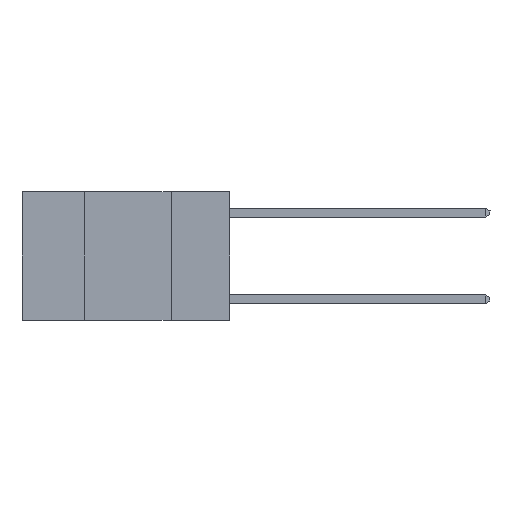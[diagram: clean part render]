
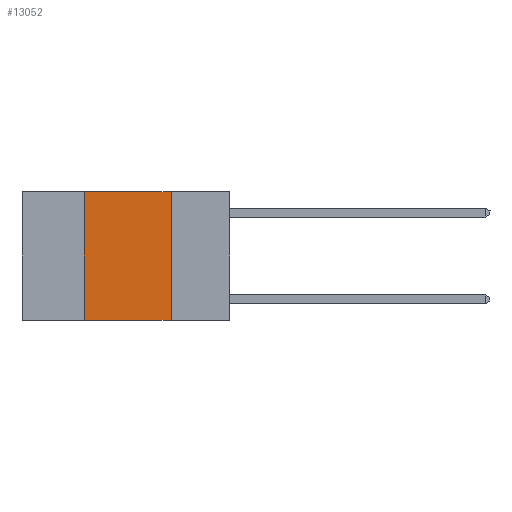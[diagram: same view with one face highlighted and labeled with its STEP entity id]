
A CAD part, left-side view. The second image highlights one B-rep face of the part: STEP entity #13052.
In plain terms, the highlighted planar face has unit normal (-1, 0, 0).
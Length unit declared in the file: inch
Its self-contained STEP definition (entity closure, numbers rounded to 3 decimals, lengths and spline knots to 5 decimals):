
#58 = VERTEX_POINT ( 'NONE', #12671 ) ;
#688 = VECTOR ( 'NONE', #11399, 39.37008 ) ;
#2218 = ORIENTED_EDGE ( 'NONE', *, *, #10114, .F. ) ;
#2657 = VERTEX_POINT ( 'NONE', #5608 ) ;
#2762 = EDGE_LOOP ( 'NONE', ( #5938, #7708, #2218, #2902 ) ) ;
#2902 = ORIENTED_EDGE ( 'NONE', *, *, #3313, .T. ) ;
#3120 = CARTESIAN_POINT ( 'NONE',  ( 0., 0.6, 0. ) ) ;
#3313 = EDGE_CURVE ( 'NONE', #58, #2657, #3340, .T. ) ;
#3340 = LINE ( 'NONE', #7370, #688 ) ;
#3396 = CARTESIAN_POINT ( 'NONE',  ( 0., 0.42, 0. ) ) ;
#4567 = CARTESIAN_POINT ( 'NONE',  ( 0., 0.42, 0. ) ) ;
#4629 = LINE ( 'NONE', #4567, #4911 ) ;
#4688 = VECTOR ( 'NONE', #6193, 39.37008 ) ;
#4911 = VECTOR ( 'NONE', #8607, 39.37008 ) ;
#5608 = CARTESIAN_POINT ( 'NONE',  ( 0., 0.17, -0.37 ) ) ;
#5899 = DIRECTION ( 'NONE',  ( 0., 0., -1. ) ) ;
#5938 = ORIENTED_EDGE ( 'NONE', *, *, #8501, .F. ) ;
#6193 = DIRECTION ( 'NONE',  ( 0., -1., 0. ) ) ;
#6664 = AXIS2_PLACEMENT_3D ( 'NONE', #3120, #7133, #5899 ) ;
#6924 = VERTEX_POINT ( 'NONE', #8530 ) ;
#7133 = DIRECTION ( 'NONE',  ( 1., 0., 0. ) ) ;
#7370 = CARTESIAN_POINT ( 'NONE',  ( 0., 0.6, -0.37 ) ) ;
#7708 = ORIENTED_EDGE ( 'NONE', *, *, #9451, .F. ) ;
#8059 = CARTESIAN_POINT ( 'NONE',  ( 0., 0.6, 0. ) ) ;
#8501 = EDGE_CURVE ( 'NONE', #6924, #2657, #11124, .T. ) ;
#8530 = CARTESIAN_POINT ( 'NONE',  ( 0., 0.17, 0. ) ) ;
#8607 = DIRECTION ( 'NONE',  ( 0., 0., 1. ) ) ;
#9120 = CARTESIAN_POINT ( 'NONE',  ( 0., 0.17, 0. ) ) ;
#9451 = EDGE_CURVE ( 'NONE', #10712, #6924, #11232, .T. ) ;
#10114 = EDGE_CURVE ( 'NONE', #58, #10712, #4629, .T. ) ;
#10204 = DIRECTION ( 'NONE',  ( 0., 0., -1. ) ) ;
#10712 = VERTEX_POINT ( 'NONE', #3396 ) ;
#11124 = LINE ( 'NONE', #9120, #12104 ) ;
#11232 = LINE ( 'NONE', #8059, #4688 ) ;
#11399 = DIRECTION ( 'NONE',  ( 0., -1., 0. ) ) ;
#12104 = VECTOR ( 'NONE', #10204, 39.37008 ) ;
#12193 = FACE_OUTER_BOUND ( 'NONE', #2762, .T. ) ;
#12258 = PLANE ( 'NONE',  #6664 ) ;
#12671 = CARTESIAN_POINT ( 'NONE',  ( 0., 0.42, -0.37 ) ) ;
#13052 = ADVANCED_FACE ( 'NONE', ( #12193 ), #12258, .F. ) ;
